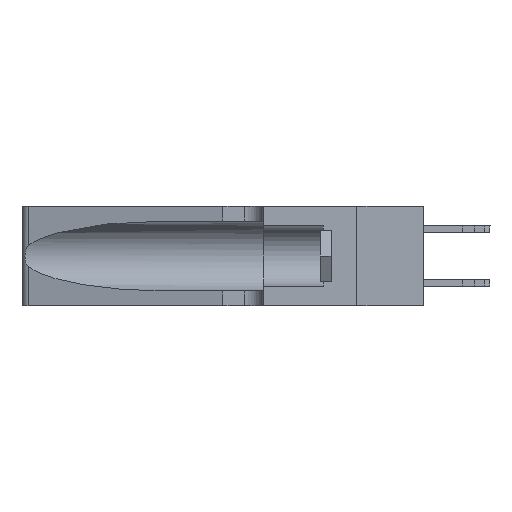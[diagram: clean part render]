
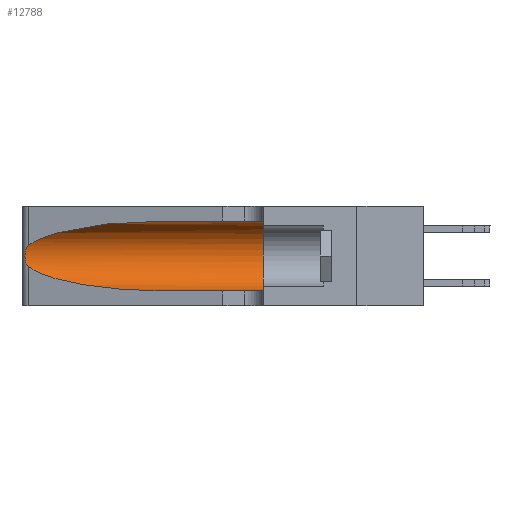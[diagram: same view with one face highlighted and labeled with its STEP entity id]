
A CAD part, left-side view. The second image highlights one B-rep face of the part: STEP entity #12788.
In plain terms, the highlighted cylindrical face has radius 3.308 mm (diameter 6.617 mm), a partial arc.
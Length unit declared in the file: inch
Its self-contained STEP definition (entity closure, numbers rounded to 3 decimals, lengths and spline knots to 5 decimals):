
#300 = VERTEX_POINT ( 'NONE', #18111 ) ;
#489 = EDGE_CURVE ( 'NONE', #27499, #1107, #850, .T. ) ;
#850 = B_SPLINE_CURVE_WITH_KNOTS ( 'NONE', 3,
 ( #7239, #21222, #4733, #1439, #31851, #1564, #22011, #14408, #30701, #11550, #3179, #6211, #33569, #8982 ),
 .UNSPECIFIED., .F., .F.,
 ( 4, 2, 2, 2, 2, 2, 4 ),
 ( 0., 0.00027, 0.00053, 0.00107, 0.0016, 0.00187, 0.00214 ),
 .UNSPECIFIED. ) ;
#1107 = VERTEX_POINT ( 'NONE', #34299 ) ;
#1439 = CARTESIAN_POINT ( 'NONE',  ( 0.25787, 1.23484, 0.2124 ) ) ;
#1564 = CARTESIAN_POINT ( 'NONE',  ( 0.26018, 1.23835, 0.19895 ) ) ;
#1826 = DIRECTION ( 'NONE',  ( 0., -1., 0. ) ) ;
#2113 = ORIENTED_EDGE ( 'NONE', *, *, #19376, .F. ) ;
#3179 = CARTESIAN_POINT ( 'NONE',  ( 0.25789, 1.23486, 0.15765 ) ) ;
#4704 = VERTEX_POINT ( 'NONE', #20272 ) ;
#4733 = CARTESIAN_POINT ( 'NONE',  ( 0.25639, 1.23184, 0.21858 ) ) ;
#5292 = DIRECTION ( 'NONE',  ( 0., -1., 0. ) ) ;
#6211 = CARTESIAN_POINT ( 'NONE',  ( 0.25639, 1.23186, 0.15144 ) ) ;
#7151 = EDGE_CURVE ( 'NONE', #300, #27499, #20077, .T. ) ;
#7239 = CARTESIAN_POINT ( 'NONE',  ( 0.25487, 1.22718, 0.22369 ) ) ;
#7253 = EDGE_LOOP ( 'NONE', ( #16607, #20933, #9054, #29358, #7623, #2113 ) ) ;
#7623 = ORIENTED_EDGE ( 'NONE', *, *, #11839, .F. ) ;
#8826 = CARTESIAN_POINT ( 'NONE',  ( 0.1305, 0.35, 0.05475 ) ) ;
#8908 = AXIS2_PLACEMENT_3D ( 'NONE', #26536, #1826, #21941 ) ;
#8918 = VERTEX_POINT ( 'NONE', #8826 ) ;
#8982 = CARTESIAN_POINT ( 'NONE',  ( 0.25487, 1.22718, 0.14631 ) ) ;
#9054 = ORIENTED_EDGE ( 'NONE', *, *, #19957, .T. ) ;
#9108 = CARTESIAN_POINT ( 'NONE',  ( 0.2373, 1.15595, 0.28018 ) ) ;
#9832 = AXIS2_PLACEMENT_3D ( 'NONE', #20168, #28030, #30828 ) ;
#11550 = CARTESIAN_POINT ( 'NONE',  ( 0.25856, 1.23593, 0.16098 ) ) ;
#11839 = EDGE_CURVE ( 'NONE', #4704, #8918, #29748, .T. ) ;
#12404 = EDGE_CURVE ( 'NONE', #22272, #8918, #13336, .T. ) ;
#12429 = FACE_OUTER_BOUND ( 'NONE', #7253, .T. ) ;
#12788 = ADVANCED_FACE ( 'NONE', ( #12429 ), #26197, .F. ) ;
#12981 = CARTESIAN_POINT ( 'NONE',  ( 0.25487, 1.22718, 0.22369 ) ) ;
#13336 = LINE ( 'NONE', #16205, #32727 ) ;
#14408 = CARTESIAN_POINT ( 'NONE',  ( 0.26075, 1.23896, 0.178 ) ) ;
#14793 = VECTOR ( 'NONE', #26806, 39.37008 ) ;
#15050 = CARTESIAN_POINT ( 'NONE',  ( 0.25487, 1.22718, 0.14631 ) ) ;
#16205 = CARTESIAN_POINT ( 'NONE',  ( 0.1305, 1.61858, 0.05475 ) ) ;
#16607 = ORIENTED_EDGE ( 'NONE', *, *, #7151, .T. ) ;
#17266 = CARTESIAN_POINT ( 'NONE',  ( 0.18966, 0.96281, 0.31525 ) ) ;
#17640 =( BOUNDED_CURVE ( )  B_SPLINE_CURVE ( 3, ( #15050, #17950, #29053, #31842 ),
 .UNSPECIFIED., .F., .F. ) 
 B_SPLINE_CURVE_WITH_KNOTS ( ( 4, 4 ),
 ( 3.44316, 4.71239 ),
 .UNSPECIFIED. ) 
 CURVE ( )  GEOMETRIC_REPRESENTATION_ITEM ( )  RATIONAL_B_SPLINE_CURVE ( ( 1., 0.87, 0.87, 1. ) ) 
 REPRESENTATION_ITEM ( '' )  );
#17950 = CARTESIAN_POINT ( 'NONE',  ( 0.2373, 1.15595, 0.08982 ) ) ;
#18111 = CARTESIAN_POINT ( 'NONE',  ( 0.1305, 0.72297, 0.31525 ) ) ;
#19376 = EDGE_CURVE ( 'NONE', #300, #4704, #31208, .T. ) ;
#19957 = EDGE_CURVE ( 'NONE', #1107, #22272, #17640, .T. ) ;
#20077 =( BOUNDED_CURVE ( )  B_SPLINE_CURVE ( 3, ( #31054, #17266, #9108, #12981 ),
 .UNSPECIFIED., .F., .T. ) 
 B_SPLINE_CURVE_WITH_KNOTS ( ( 4, 4 ),
 ( 1.5708, 2.84003 ),
 .UNSPECIFIED. ) 
 CURVE ( )  GEOMETRIC_REPRESENTATION_ITEM ( )  RATIONAL_B_SPLINE_CURVE ( ( 1., 0.87, 0.87, 1. ) ) 
 REPRESENTATION_ITEM ( '' )  );
#20168 = CARTESIAN_POINT ( 'NONE',  ( 0.1305, 0.35, 0.185 ) ) ;
#20272 = CARTESIAN_POINT ( 'NONE',  ( 0.1305, 0.35, 0.31525 ) ) ;
#20933 = ORIENTED_EDGE ( 'NONE', *, *, #489, .T. ) ;
#21222 = CARTESIAN_POINT ( 'NONE',  ( 0.25555, 1.22994, 0.2215 ) ) ;
#21264 = CARTESIAN_POINT ( 'NONE',  ( 0.1305, 1.61858, 0.31525 ) ) ;
#21941 = DIRECTION ( 'NONE',  ( 0., 0., -1. ) ) ;
#22011 = CARTESIAN_POINT ( 'NONE',  ( 0.26075, 1.23896, 0.19203 ) ) ;
#22272 = VERTEX_POINT ( 'NONE', #32628 ) ;
#26197 = CYLINDRICAL_SURFACE ( 'NONE', #8908, 0.13025 ) ;
#26536 = CARTESIAN_POINT ( 'NONE',  ( 0.1305, 1.61858, 0.185 ) ) ;
#26806 = DIRECTION ( 'NONE',  ( 0., -1., 0. ) ) ;
#27499 = VERTEX_POINT ( 'NONE', #35016 ) ;
#28030 = DIRECTION ( 'NONE',  ( 0., 1., 0. ) ) ;
#29053 = CARTESIAN_POINT ( 'NONE',  ( 0.18966, 0.96281, 0.05475 ) ) ;
#29358 = ORIENTED_EDGE ( 'NONE', *, *, #12404, .T. ) ;
#29748 = CIRCLE ( 'NONE', #9832, 0.13025 ) ;
#30701 = CARTESIAN_POINT ( 'NONE',  ( 0.26017, 1.23833, 0.17102 ) ) ;
#30828 = DIRECTION ( 'NONE',  ( 0., 0., 1. ) ) ;
#31054 = CARTESIAN_POINT ( 'NONE',  ( 0.1305, 0.72297, 0.31525 ) ) ;
#31208 = LINE ( 'NONE', #21264, #14793 ) ;
#31842 = CARTESIAN_POINT ( 'NONE',  ( 0.1305, 0.72297, 0.05475 ) ) ;
#31851 = CARTESIAN_POINT ( 'NONE',  ( 0.25854, 1.2359, 0.20912 ) ) ;
#32628 = CARTESIAN_POINT ( 'NONE',  ( 0.1305, 0.72297, 0.05475 ) ) ;
#32727 = VECTOR ( 'NONE', #5292, 39.37008 ) ;
#33569 = CARTESIAN_POINT ( 'NONE',  ( 0.25555, 1.22993, 0.14849 ) ) ;
#34299 = CARTESIAN_POINT ( 'NONE',  ( 0.25487, 1.22718, 0.14631 ) ) ;
#35016 = CARTESIAN_POINT ( 'NONE',  ( 0.25487, 1.22718, 0.22369 ) ) ;
